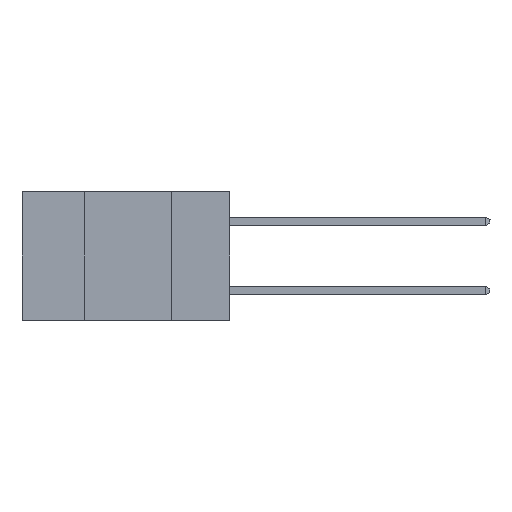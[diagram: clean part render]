
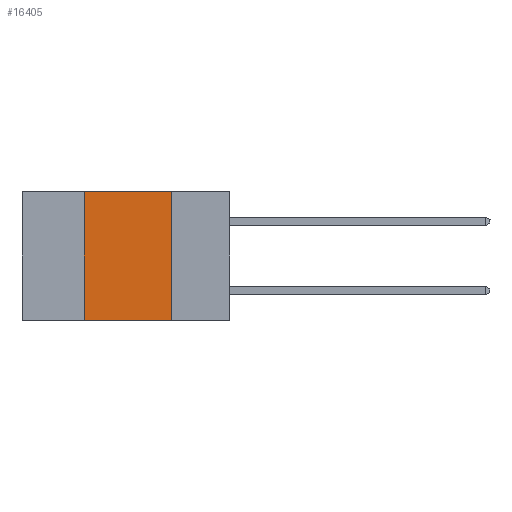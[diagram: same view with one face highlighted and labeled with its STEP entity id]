
A CAD part, left-side view. The second image highlights one B-rep face of the part: STEP entity #16405.
In plain terms, the highlighted planar face has unit normal (-1, 0, 0).
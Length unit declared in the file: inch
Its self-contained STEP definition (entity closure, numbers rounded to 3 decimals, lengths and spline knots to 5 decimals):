
#109 = DIRECTION ( 'NONE',  ( 0., 0., -1. ) ) ;
#373 = VECTOR ( 'NONE', #22353, 39.37008 ) ;
#1251 = CARTESIAN_POINT ( 'NONE',  ( 0., 0.42, -0.37 ) ) ;
#1528 = VECTOR ( 'NONE', #1960, 39.37008 ) ;
#1960 = DIRECTION ( 'NONE',  ( 0., -1., 0. ) ) ;
#2063 = LINE ( 'NONE', #2192, #18332 ) ;
#2192 = CARTESIAN_POINT ( 'NONE',  ( 0., 0.17, -0.37 ) ) ;
#2471 = VERTEX_POINT ( 'NONE', #8317 ) ;
#2701 = EDGE_LOOP ( 'NONE', ( #16533, #14170, #23149, #7395 ) ) ;
#3720 = FACE_OUTER_BOUND ( 'NONE', #2701, .T. ) ;
#5225 = VERTEX_POINT ( 'NONE', #24153 ) ;
#6225 = EDGE_CURVE ( 'NONE', #2471, #17532, #22140, .T. ) ;
#6951 = LINE ( 'NONE', #8886, #13358 ) ;
#7395 = ORIENTED_EDGE ( 'NONE', *, *, #22100, .T. ) ;
#7696 = CARTESIAN_POINT ( 'NONE',  ( 0., 0.42, -0.37 ) ) ;
#8150 = EDGE_CURVE ( 'NONE', #22355, #2471, #13764, .T. ) ;
#8317 = CARTESIAN_POINT ( 'NONE',  ( 0., 0.42, 0. ) ) ;
#8886 = CARTESIAN_POINT ( 'NONE',  ( 0., 0.6, -0.37 ) ) ;
#11624 = CARTESIAN_POINT ( 'NONE',  ( 0., 0.6, 0. ) ) ;
#12134 = DIRECTION ( 'NONE',  ( 0., 0., -1. ) ) ;
#13358 = VECTOR ( 'NONE', #25764, 39.37008 ) ;
#13764 = LINE ( 'NONE', #7696, #373 ) ;
#14170 = ORIENTED_EDGE ( 'NONE', *, *, #6225, .F. ) ;
#16405 = ADVANCED_FACE ( 'NONE', ( #3720 ), #20724, .F. ) ;
#16533 = ORIENTED_EDGE ( 'NONE', *, *, #24293, .F. ) ;
#17532 = VERTEX_POINT ( 'NONE', #24928 ) ;
#18332 = VECTOR ( 'NONE', #109, 39.37008 ) ;
#20317 = AXIS2_PLACEMENT_3D ( 'NONE', #24460, #26820, #12134 ) ;
#20724 = PLANE ( 'NONE',  #20317 ) ;
#22100 = EDGE_CURVE ( 'NONE', #22355, #5225, #6951, .T. ) ;
#22140 = LINE ( 'NONE', #11624, #1528 ) ;
#22353 = DIRECTION ( 'NONE',  ( 0., 0., 1. ) ) ;
#22355 = VERTEX_POINT ( 'NONE', #1251 ) ;
#23149 = ORIENTED_EDGE ( 'NONE', *, *, #8150, .F. ) ;
#24153 = CARTESIAN_POINT ( 'NONE',  ( 0., 0.17, -0.37 ) ) ;
#24293 = EDGE_CURVE ( 'NONE', #17532, #5225, #2063, .T. ) ;
#24460 = CARTESIAN_POINT ( 'NONE',  ( 0., 0.6, 0. ) ) ;
#24928 = CARTESIAN_POINT ( 'NONE',  ( 0., 0.17, 0. ) ) ;
#25764 = DIRECTION ( 'NONE',  ( 0., -1., 0. ) ) ;
#26820 = DIRECTION ( 'NONE',  ( 1., 0., 0. ) ) ;
